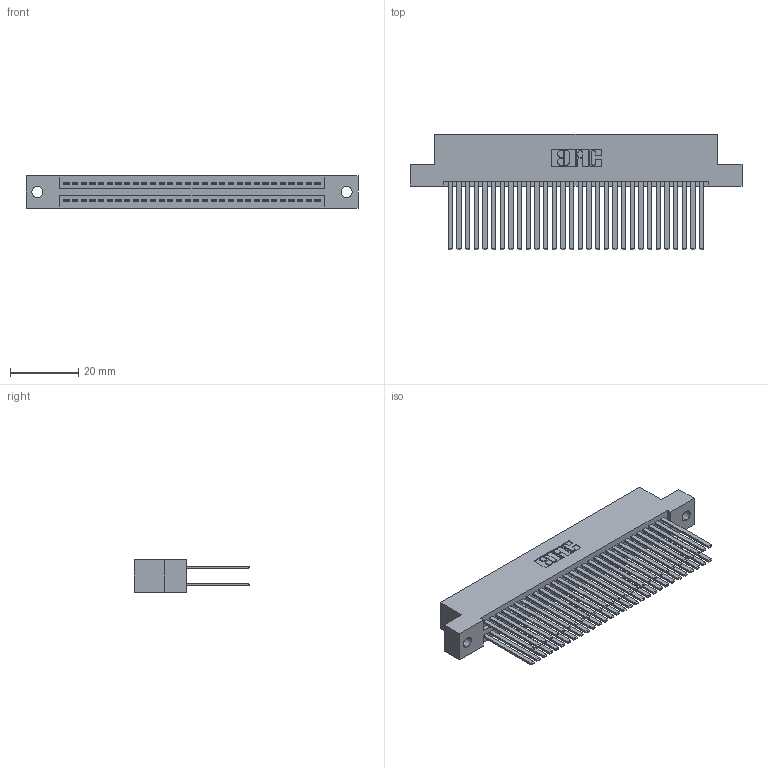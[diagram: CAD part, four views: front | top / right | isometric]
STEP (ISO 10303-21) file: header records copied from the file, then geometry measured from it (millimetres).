
FILE_DESCRIPTION (( 'STEP AP203' ), '1' );
FILE_NAME ('395-060-544-202.STEP', '2019-10-23T14:24:20', ( '' ), ( '' ), 'SwSTEP 2.0', 'SolidWorks 2016', '' );
FILE_SCHEMA (( 'CONFIG_CONTROL_DESIGN' ));
Length unit declared in the file: inch
Products named in the file (3): 345 Part_Flush Mounting Lugs - 0.128 Dia; 345-292-001_345-293-144; 395-060-544-202
Assembly tree (61 placements, depth 2):
  395-060-544-202
    345 Part_Flush Mounting Lugs - 0.128 Dia
    345-292-001_345-293-144  x60
Bounding box: 97.41 x 33.96 x 9.4 mm (x, y, z)
Volume: 10155.4 mm3; surface area: 16971.4 mm2
Topology: 61 solids, 61 shells, 2766 faces, 8201 edges, 5386 vertices
Faces by surface type: plane 1820, cylinder 946
Entity records: 24973 total; most frequent: CARTESIAN_POINT 4196, ORIENTED_EDGE 4130, DIRECTION 3713, EDGE_CURVE 2065, LINE 1817, VECTOR 1817, VERTEX_POINT 1374, AXIS2_PLACEMENT_3D 948
